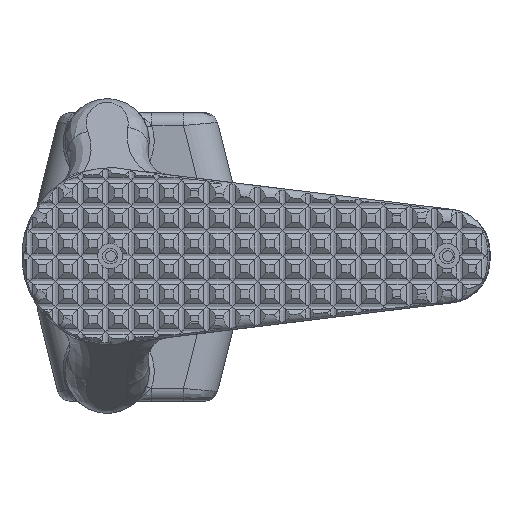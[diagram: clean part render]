
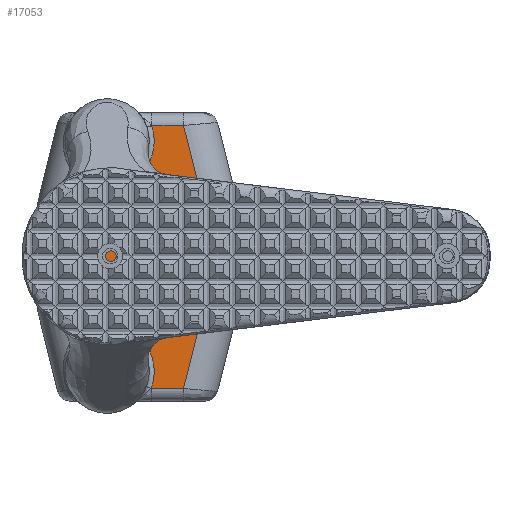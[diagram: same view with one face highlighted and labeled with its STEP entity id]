
A CAD part, left-side view. The second image highlights one B-rep face of the part: STEP entity #17053.
In plain terms, the highlighted planar face has unit normal (-1, 0, 0).
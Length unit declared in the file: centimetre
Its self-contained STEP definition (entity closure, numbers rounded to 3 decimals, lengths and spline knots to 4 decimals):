
#1317=LINE($,#31928,#2730);
#1334=LINE($,#32122,#2747);
#1336=LINE($,#32222,#2749);
#1355=LINE($,#32509,#2768);
#1364=LINE($,#32645,#2777);
#1366=LINE($,#32736,#2779);
#1461=LINE($,#33741,#2874);
#1462=LINE($,#33742,#2875);
#2730=VECTOR($,#22403,0.7545);
#2747=VECTOR($,#22458,1.8472);
#2749=VECTOR($,#22484,0.7297);
#2768=VECTOR($,#22555,0.7709);
#2777=VECTOR($,#22594,0.6915);
#2779=VECTOR($,#22620,1.8472);
#2874=VECTOR($,#22929,2.3116);
#2875=VECTOR($,#22930,2.6563);
#3762=PLANE($,#18592);
#5630=FACE_OUTER_BOUND($,#6725,.T.);
#6725=EDGE_LOOP($,(#15586,#15587,#15588,#15589,#15590,#15591,#15592,#15593,
#15594,#15595));
#7047=CIRCLE($,#18589,1.12);
#7048=CIRCLE($,#18591,1.12);
#8259=VERTEX_POINT($,#31919);
#8261=VERTEX_POINT($,#31926);
#8284=VERTEX_POINT($,#32121);
#8288=VERTEX_POINT($,#32207);
#8290=VERTEX_POINT($,#32220);
#8320=VERTEX_POINT($,#32481);
#8322=VERTEX_POINT($,#32507);
#8336=VERTEX_POINT($,#32635);
#8337=VERTEX_POINT($,#32644);
#8342=VERTEX_POINT($,#32734);
#10549=EDGE_CURVE($,#8261,#8259,#1317,.T.);
#10585=EDGE_CURVE($,#8259,#8284,#1334,.T.);
#10598=EDGE_CURVE($,#8290,#8288,#1336,.T.);
#10644=EDGE_CURVE($,#8322,#8320,#1355,.T.);
#10666=EDGE_CURVE($,#8336,#8337,#1364,.T.);
#10678=EDGE_CURVE($,#8342,#8322,#1366,.T.);
#10868=EDGE_CURVE($,#8288,#8261,#7047,.T.);
#10869=EDGE_CURVE($,#8320,#8336,#7048,.T.);
#10870=EDGE_CURVE($,#8337,#8290,#1461,.T.);
#10871=EDGE_CURVE($,#8284,#8342,#1462,.T.);
#15586=ORIENTED_EDGE($,*,*,#10868,.F.);
#15587=ORIENTED_EDGE($,*,*,#10598,.F.);
#15588=ORIENTED_EDGE($,*,*,#10870,.F.);
#15589=ORIENTED_EDGE($,*,*,#10666,.F.);
#15590=ORIENTED_EDGE($,*,*,#10869,.F.);
#15591=ORIENTED_EDGE($,*,*,#10644,.F.);
#15592=ORIENTED_EDGE($,*,*,#10678,.F.);
#15593=ORIENTED_EDGE($,*,*,#10871,.F.);
#15594=ORIENTED_EDGE($,*,*,#10585,.F.);
#15595=ORIENTED_EDGE($,*,*,#10549,.F.);
#17053=ADVANCED_FACE($,(#5630),#3762,.F.);
#18589=AXIS2_PLACEMENT_3D($,#33737,#22921,#22922);
#18591=AXIS2_PLACEMENT_3D($,#33739,#22925,#22926);
#18592=AXIS2_PLACEMENT_3D($,#33740,#22927,#22928);
#22403=DIRECTION($,(0.,-1.,0.));
#22458=DIRECTION($,(0.,-0.243,-0.97));
#22484=DIRECTION($,(0.,-0.243,0.97));
#22555=DIRECTION($,(0.,1.,0.));
#22594=DIRECTION($,(0.,0.243,0.97));
#22620=DIRECTION($,(0.,0.243,-0.97));
#22921=DIRECTION('center_axis',(-1.,0.,0.));
#22922=DIRECTION('ref_axis',(0.,-0.582,
-0.813));
#22925=DIRECTION('center_axis',(-1.,0.,0.));
#22926=DIRECTION('ref_axis',(0.,-0.596,0.803));
#22927=DIRECTION('center_axis',(1.,0.,0.));
#22928=DIRECTION('ref_axis',(0.,0.,1.));
#22929=DIRECTION($,(0.,0.,1.));
#22930=DIRECTION($,(0.,0.,-1.));
#31919=CARTESIAN_POINT('',(-24.4146,1.5148,23.2209));
#31926=CARTESIAN_POINT('',(-24.4146,2.2693,23.2209));
#31928=CARTESIAN_POINT($,(-24.4146,3.754,23.2209));
#32121=CARTESIAN_POINT('',(-24.4146,1.0667,21.4288));
#32122=CARTESIAN_POINT($,(-24.4146,0.963,21.0138));
#32207=CARTESIAN_POINT('',(-24.4146,4.0074,21.9644));
#32220=CARTESIAN_POINT('',(-24.4146,4.1843,21.2565));
#32222=CARTESIAN_POINT($,(-24.4146,4.3875,20.4437));
#32481=CARTESIAN_POINT('',(-24.4146,2.2856,16.9804));
#32507=CARTESIAN_POINT('',(-24.4146,1.5148,16.9804));
#32509=CARTESIAN_POINT($,(-24.4146,3.754,16.9804));
#32635=CARTESIAN_POINT('',(-24.4146,4.0166,18.274));
#32644=CARTESIAN_POINT('',(-24.4146,4.1843,18.9449));
#32645=CARTESIAN_POINT($,(-24.4146,3.7448,17.1866));
#32734=CARTESIAN_POINT('',(-24.4146,1.0667,18.7725));
#32736=CARTESIAN_POINT($,(-24.4146,1.6058,16.6164));
#33737=CARTESIAN_POINT('Origin',(-24.4146,3.3277,22.8546));
#33739=CARTESIAN_POINT('Origin',(-24.4146,3.3277,17.391));
#33740=CARTESIAN_POINT('Origin',(-24.4146,4.3055,17.3689));
#33741=CARTESIAN_POINT($,(-24.4146,4.1843,18.7345));
#33742=CARTESIAN_POINT($,(-24.4146,1.0667,18.7345));
